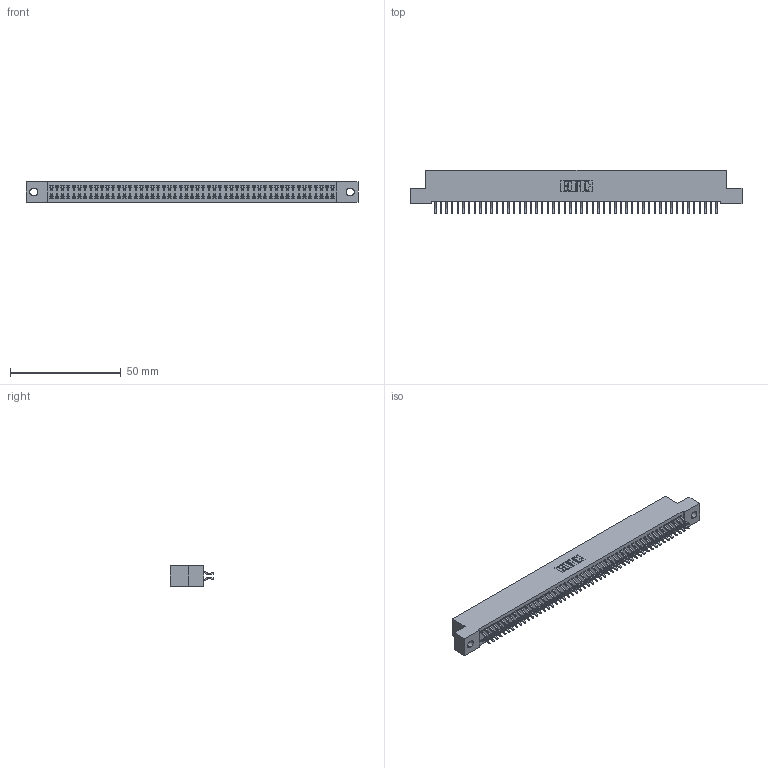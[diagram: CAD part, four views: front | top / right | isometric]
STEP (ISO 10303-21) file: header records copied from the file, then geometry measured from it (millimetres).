
FILE_DESCRIPTION (( 'STEP AP203' ), '1' );
FILE_NAME ('392-102-556-202.STEP', '2018-08-18T19:08:30', ( '' ), ( '' ), 'SwSTEP 2.0', 'SolidWorks 2016', '' );
FILE_SCHEMA (( 'CONFIG_CONTROL_DESIGN' ));
Length unit declared in the file: inch
Products named in the file (3): 345-292-001_556 Tail; 392-102-556-202; 342 Part_.128 Slot
Assembly tree (103 placements, depth 2):
  392-102-556-202
    342 Part_.128 Slot
    345-292-001_556 Tail  x102
Bounding box: 149.86 x 19.58 x 9.4 mm (x, y, z)
Volume: 13452.8 mm3; surface area: 21780 mm2
Topology: 103 solids, 103 shells, 6030 faces, 17957 edges, 11834 vertices
Faces by surface type: plane 4150, cylinder 1880
Entity records: 31869 total; most frequent: CARTESIAN_POINT 5286, ORIENTED_EDGE 5210, DIRECTION 4489, EDGE_CURVE 2605, LINE 2469, VECTOR 2469, VERTEX_POINT 1734, AXIS2_PLACEMENT_3D 1010
